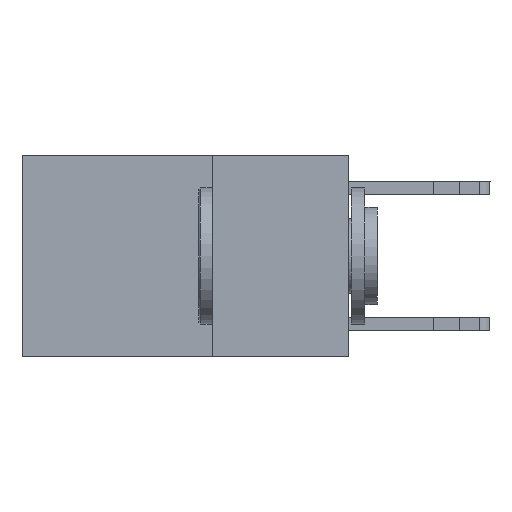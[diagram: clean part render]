
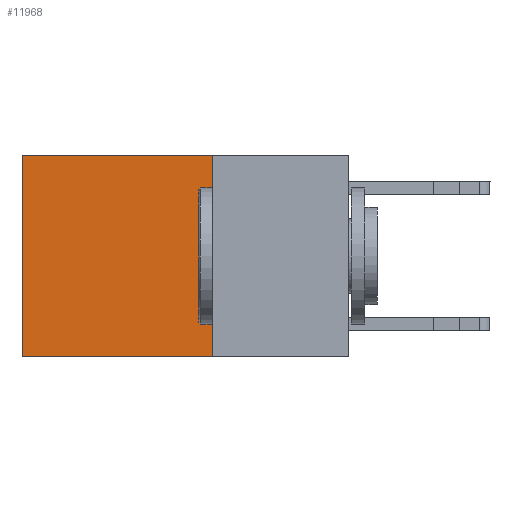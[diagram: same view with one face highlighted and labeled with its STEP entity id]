
A CAD part, left-side view. The second image highlights one B-rep face of the part: STEP entity #11968.
In plain terms, the highlighted planar face has unit normal (-1, 0, 0).
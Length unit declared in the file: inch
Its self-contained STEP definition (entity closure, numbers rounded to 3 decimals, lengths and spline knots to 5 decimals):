
#47 = CARTESIAN_POINT ( 'NONE',  ( 0.2625, 0.25, 0. ) ) ;
#571 = FACE_OUTER_BOUND ( 'NONE', #13739, .T. ) ;
#651 = LINE ( 'NONE', #10485, #12025 ) ;
#757 = CARTESIAN_POINT ( 'NONE',  ( 0.2625, 0.6, 0. ) ) ;
#1066 = DIRECTION ( 'NONE',  ( 0., 1., 0. ) ) ;
#1470 = CARTESIAN_POINT ( 'NONE',  ( 0.2625, 0.6, -0.37 ) ) ;
#1801 = LINE ( 'NONE', #9372, #9135 ) ;
#2471 = DIRECTION ( 'NONE',  ( 0., 0., -1. ) ) ;
#2768 = VECTOR ( 'NONE', #1066, 39.37008 ) ;
#4963 = VERTEX_POINT ( 'NONE', #757 ) ;
#5024 = EDGE_CURVE ( 'NONE', #9215, #12656, #1801, .T. ) ;
#5126 = DIRECTION ( 'NONE',  ( 0., 0., -1. ) ) ;
#5316 = CARTESIAN_POINT ( 'NONE',  ( 0.2625, 0.25, -0.37 ) ) ;
#5500 = AXIS2_PLACEMENT_3D ( 'NONE', #12177, #5824, #2471 ) ;
#5690 = VECTOR ( 'NONE', #6033, 39.37008 ) ;
#5824 = DIRECTION ( 'NONE',  ( 1., 0., 0. ) ) ;
#6033 = DIRECTION ( 'NONE',  ( 0., 1., 0. ) ) ;
#6975 = CARTESIAN_POINT ( 'NONE',  ( 0.2625, 0.25, 0. ) ) ;
#7419 = VERTEX_POINT ( 'NONE', #1470 ) ;
#7562 = ORIENTED_EDGE ( 'NONE', *, *, #10043, .T. ) ;
#8369 = ORIENTED_EDGE ( 'NONE', *, *, #5024, .F. ) ;
#8590 = LINE ( 'NONE', #47, #2768 ) ;
#8912 = EDGE_CURVE ( 'NONE', #12656, #7419, #12859, .T. ) ;
#9135 = VECTOR ( 'NONE', #13679, 39.37008 ) ;
#9170 = CARTESIAN_POINT ( 'NONE',  ( 0.2625, 0.25, -0.37 ) ) ;
#9215 = VERTEX_POINT ( 'NONE', #6975 ) ;
#9372 = CARTESIAN_POINT ( 'NONE',  ( 0.2625, 0.25, 0. ) ) ;
#10043 = EDGE_CURVE ( 'NONE', #9215, #4963, #8590, .T. ) ;
#10485 = CARTESIAN_POINT ( 'NONE',  ( 0.2625, 0.6, 0. ) ) ;
#11741 = EDGE_CURVE ( 'NONE', #4963, #7419, #651, .T. ) ;
#11968 = ADVANCED_FACE ( 'NONE', ( #571 ), #12117, .F. ) ;
#12025 = VECTOR ( 'NONE', #5126, 39.37008 ) ;
#12069 = ORIENTED_EDGE ( 'NONE', *, *, #11741, .T. ) ;
#12117 = PLANE ( 'NONE',  #5500 ) ;
#12177 = CARTESIAN_POINT ( 'NONE',  ( 0.2625, 0.25, 0. ) ) ;
#12656 = VERTEX_POINT ( 'NONE', #9170 ) ;
#12859 = LINE ( 'NONE', #5316, #5690 ) ;
#13539 = ORIENTED_EDGE ( 'NONE', *, *, #8912, .F. ) ;
#13679 = DIRECTION ( 'NONE',  ( 0., 0., -1. ) ) ;
#13739 = EDGE_LOOP ( 'NONE', ( #12069, #13539, #8369, #7562 ) ) ;
